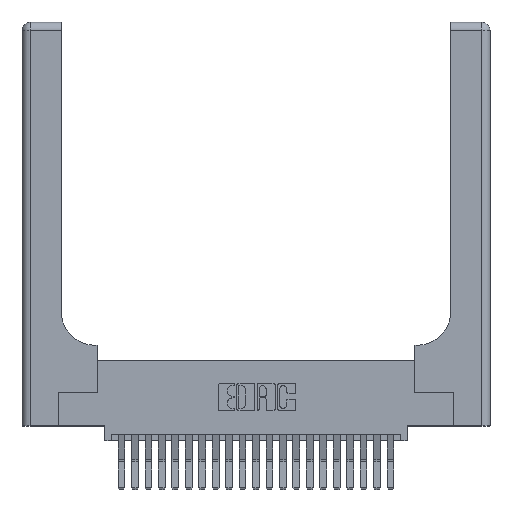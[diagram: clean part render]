
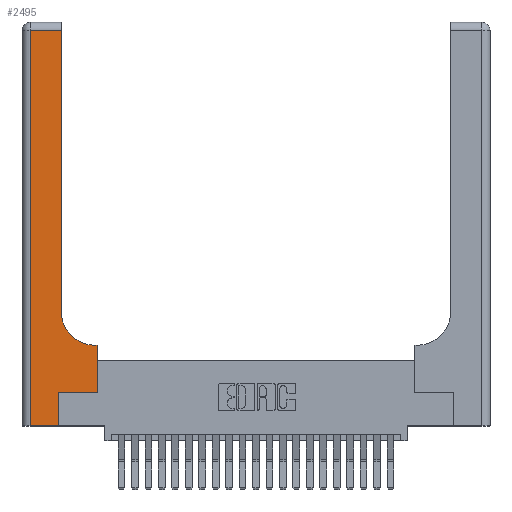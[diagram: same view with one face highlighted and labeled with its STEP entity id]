
A CAD part, top view. The second image highlights one B-rep face of the part: STEP entity #2495.
In plain terms, the highlighted planar face has unit normal (0, 0, 1).
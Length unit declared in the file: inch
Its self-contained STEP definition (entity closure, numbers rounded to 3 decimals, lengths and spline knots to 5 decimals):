
#167 = CARTESIAN_POINT ( 'NONE',  ( 0.2915, 0.85, 0.37 ) ) ;
#323 = VERTEX_POINT ( 'NONE', #19905 ) ;
#333 = ORIENTED_EDGE ( 'NONE', *, *, #7674, .T. ) ;
#1396 = DIRECTION ( 'NONE',  ( 0., -1., 0. ) ) ;
#1872 = VECTOR ( 'NONE', #1396, 39.37008 ) ;
#1948 = VERTEX_POINT ( 'NONE', #24007 ) ;
#2183 = VERTEX_POINT ( 'NONE', #18785 ) ;
#2495 = ADVANCED_FACE ( 'NONE', ( #6271 ), #17165, .F. ) ;
#3350 = DIRECTION ( 'NONE',  ( 0., 0., -1. ) ) ;
#3523 = LINE ( 'NONE', #17016, #4693 ) ;
#3583 = LINE ( 'NONE', #6788, #18156 ) ;
#4173 = DIRECTION ( 'NONE',  ( -1., 0., 0. ) ) ;
#4340 = CARTESIAN_POINT ( 'NONE',  ( 0., 2.94, 0.37 ) ) ;
#4640 = DIRECTION ( 'NONE',  ( 0., 1., 0. ) ) ;
#4693 = VECTOR ( 'NONE', #5524, 39.37008 ) ;
#4931 = VERTEX_POINT ( 'NONE', #15026 ) ;
#5069 = CARTESIAN_POINT ( 'NONE',  ( 0.06, 3., 0.37 ) ) ;
#5494 = EDGE_CURVE ( 'NONE', #21550, #2183, #14835, .T. ) ;
#5524 = DIRECTION ( 'NONE',  ( 0., 1., 0. ) ) ;
#5699 = DIRECTION ( 'NONE',  ( -1., 0., 0. ) ) ;
#5780 = ORIENTED_EDGE ( 'NONE', *, *, #7218, .T. ) ;
#5886 = VECTOR ( 'NONE', #20844, 39.37008 ) ;
#6114 = LINE ( 'NONE', #4340, #19037 ) ;
#6271 = FACE_OUTER_BOUND ( 'NONE', #8845, .T. ) ;
#6788 = CARTESIAN_POINT ( 'NONE',  ( 0.5585, 0.25, 0.37 ) ) ;
#7218 = EDGE_CURVE ( 'NONE', #1948, #19791, #19904, .T. ) ;
#7425 = CARTESIAN_POINT ( 'NONE',  ( 0.2915, 0.6, 0.37 ) ) ;
#7616 = EDGE_CURVE ( 'NONE', #19791, #9956, #3523, .T. ) ;
#7647 = VECTOR ( 'NONE', #12827, 39.37008 ) ;
#7674 = EDGE_CURVE ( 'NONE', #22766, #1948, #19005, .T. ) ;
#8539 = ORIENTED_EDGE ( 'NONE', *, *, #5494, .T. ) ;
#8581 = CARTESIAN_POINT ( 'NONE',  ( 0., 0., 0.37 ) ) ;
#8845 = EDGE_LOOP ( 'NONE', ( #11364, #13601, #24519, #10495, #8539, #17779, #10810, #333, #5780 ) ) ;
#8999 = VECTOR ( 'NONE', #12804, 39.37008 ) ;
#9956 = VERTEX_POINT ( 'NONE', #17176 ) ;
#10495 = ORIENTED_EDGE ( 'NONE', *, *, #21914, .T. ) ;
#10666 = DIRECTION ( 'NONE',  ( 1., 0., 0. ) ) ;
#10810 = ORIENTED_EDGE ( 'NONE', *, *, #18251, .T. ) ;
#11154 = VERTEX_POINT ( 'NONE', #21837 ) ;
#11364 = ORIENTED_EDGE ( 'NONE', *, *, #7616, .T. ) ;
#12074 = VECTOR ( 'NONE', #10666, 39.37008 ) ;
#12804 = DIRECTION ( 'NONE',  ( 1., 0., 0. ) ) ;
#12827 = DIRECTION ( 'NONE',  ( 0., 1., 0. ) ) ;
#12852 = DIRECTION ( 'NONE',  ( 1., 0., 0. ) ) ;
#13274 = CARTESIAN_POINT ( 'NONE',  ( 0.269, 0., 0.37 ) ) ;
#13601 = ORIENTED_EDGE ( 'NONE', *, *, #18171, .T. ) ;
#14078 = LINE ( 'NONE', #24265, #8999 ) ;
#14156 = LINE ( 'NONE', #8581, #12074 ) ;
#14355 = CARTESIAN_POINT ( 'NONE',  ( 0., 3., 0.37 ) ) ;
#14835 = LINE ( 'NONE', #20404, #7647 ) ;
#15026 = CARTESIAN_POINT ( 'NONE',  ( 0.5585, 0.25, 0.37 ) ) ;
#16396 = EDGE_CURVE ( 'NONE', #11154, #323, #21239, .T. ) ;
#16535 = CARTESIAN_POINT ( 'NONE',  ( 0.5415, 0.85, 0.37 ) ) ;
#16545 = EDGE_CURVE ( 'NONE', #2183, #4931, #14078, .T. ) ;
#17016 = CARTESIAN_POINT ( 'NONE',  ( 0.2915, 3., 0.37 ) ) ;
#17165 = PLANE ( 'NONE',  #18158 ) ;
#17176 = CARTESIAN_POINT ( 'NONE',  ( 0.2915, 2.94, 0.37 ) ) ;
#17779 = ORIENTED_EDGE ( 'NONE', *, *, #16545, .T. ) ;
#18156 = VECTOR ( 'NONE', #4640, 39.37008 ) ;
#18158 = AXIS2_PLACEMENT_3D ( 'NONE', #14355, #3350, #5699 ) ;
#18171 = EDGE_CURVE ( 'NONE', #9956, #11154, #6114, .T. ) ;
#18251 = EDGE_CURVE ( 'NONE', #4931, #22766, #3583, .T. ) ;
#18424 = DIRECTION ( 'NONE',  ( 0., 0., -1. ) ) ;
#18785 = CARTESIAN_POINT ( 'NONE',  ( 0.269, 0.25, 0.37 ) ) ;
#19005 = LINE ( 'NONE', #7425, #5886 ) ;
#19037 = VECTOR ( 'NONE', #4173, 39.37008 ) ;
#19338 = AXIS2_PLACEMENT_3D ( 'NONE', #16535, #18424, #12852 ) ;
#19791 = VERTEX_POINT ( 'NONE', #167 ) ;
#19904 = CIRCLE ( 'NONE', #19338, 0.25 ) ;
#19905 = CARTESIAN_POINT ( 'NONE',  ( 0.06, 0., 0.37 ) ) ;
#20404 = CARTESIAN_POINT ( 'NONE',  ( 0.269, 0., 0.37 ) ) ;
#20844 = DIRECTION ( 'NONE',  ( -1., 0., 0. ) ) ;
#21239 = LINE ( 'NONE', #5069, #1872 ) ;
#21550 = VERTEX_POINT ( 'NONE', #13274 ) ;
#21837 = CARTESIAN_POINT ( 'NONE',  ( 0.06, 2.94, 0.37 ) ) ;
#21914 = EDGE_CURVE ( 'NONE', #323, #21550, #14156, .T. ) ;
#22645 = CARTESIAN_POINT ( 'NONE',  ( 0.5585, 0.6, 0.37 ) ) ;
#22766 = VERTEX_POINT ( 'NONE', #22645 ) ;
#24007 = CARTESIAN_POINT ( 'NONE',  ( 0.5415, 0.6, 0.37 ) ) ;
#24265 = CARTESIAN_POINT ( 'NONE',  ( 0.269, 0.25, 0.37 ) ) ;
#24519 = ORIENTED_EDGE ( 'NONE', *, *, #16396, .T. ) ;
